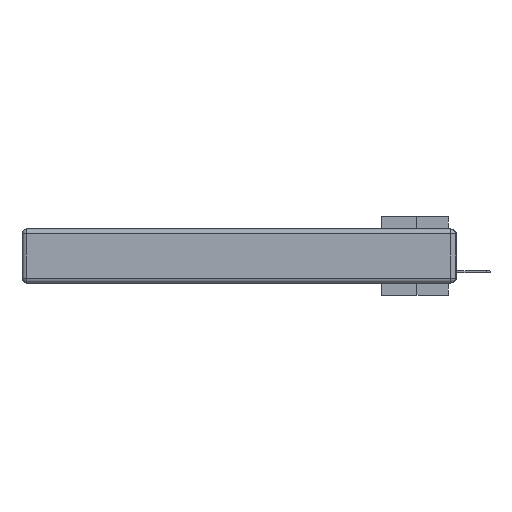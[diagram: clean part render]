
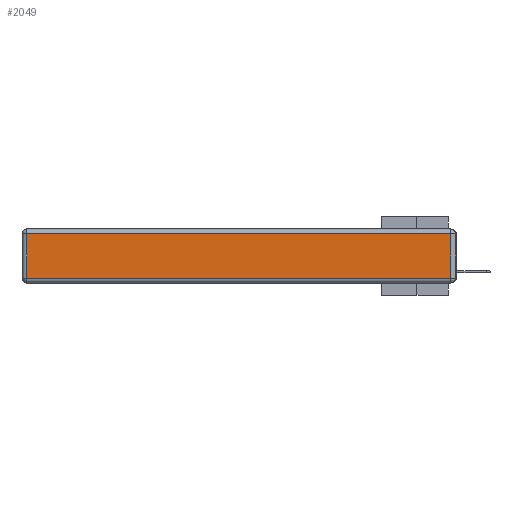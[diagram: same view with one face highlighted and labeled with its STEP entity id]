
A CAD part, left-side view. The second image highlights one B-rep face of the part: STEP entity #2049.
In plain terms, the highlighted planar face has unit normal (-1, 0, 0).
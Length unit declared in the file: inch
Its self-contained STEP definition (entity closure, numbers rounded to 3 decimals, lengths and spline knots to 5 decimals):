
#412 = DIRECTION ( 'NONE',  ( 0., 1., 0. ) ) ;
#1470 = LINE ( 'NONE', #4360, #27124 ) ;
#2049 = ADVANCED_FACE ( 'NONE', ( #32304 ), #18576, .T. ) ;
#3308 = CARTESIAN_POINT ( 'NONE',  ( 0., 2.75, -0.03 ) ) ;
#3401 = EDGE_CURVE ( 'NONE', #28576, #4793, #19665, .T. ) ;
#3579 = ORIENTED_EDGE ( 'NONE', *, *, #27160, .T. ) ;
#4360 = CARTESIAN_POINT ( 'NONE',  ( 0., 0.03, -0.343 ) ) ;
#4760 = CARTESIAN_POINT ( 'NONE',  ( 0., 0., -0.343 ) ) ;
#4793 = VERTEX_POINT ( 'NONE', #31206 ) ;
#6296 = EDGE_LOOP ( 'NONE', ( #3579, #31972, #23948, #17281 ) ) ;
#6326 = DIRECTION ( 'NONE',  ( 0., 0., 1. ) ) ;
#8368 = CARTESIAN_POINT ( 'NONE',  ( 0., 2.72, -0.313 ) ) ;
#8478 = EDGE_CURVE ( 'NONE', #4793, #15131, #19443, .T. ) ;
#9550 = CARTESIAN_POINT ( 'NONE',  ( 0., 0., -0.313 ) ) ;
#13141 = DIRECTION ( 'NONE',  ( -1., 0., 0. ) ) ;
#13359 = VERTEX_POINT ( 'NONE', #27454 ) ;
#15131 = VERTEX_POINT ( 'NONE', #8368 ) ;
#15206 = DIRECTION ( 'NONE',  ( 0., -1., 0. ) ) ;
#15406 = VECTOR ( 'NONE', #33001, 39.37008 ) ;
#17281 = ORIENTED_EDGE ( 'NONE', *, *, #8478, .T. ) ;
#18576 = PLANE ( 'NONE',  #34975 ) ;
#18721 = CARTESIAN_POINT ( 'NONE',  ( 0., 2.72, -0.343 ) ) ;
#19443 = LINE ( 'NONE', #18721, #15406 ) ;
#19665 = LINE ( 'NONE', #3308, #25637 ) ;
#20035 = VECTOR ( 'NONE', #15206, 39.37008 ) ;
#21422 = DIRECTION ( 'NONE',  ( 0., 0., 1. ) ) ;
#23948 = ORIENTED_EDGE ( 'NONE', *, *, #3401, .T. ) ;
#25637 = VECTOR ( 'NONE', #412, 39.37008 ) ;
#25700 = LINE ( 'NONE', #9550, #20035 ) ;
#27124 = VECTOR ( 'NONE', #21422, 39.37008 ) ;
#27153 = CARTESIAN_POINT ( 'NONE',  ( 0., 0.03, -0.03 ) ) ;
#27160 = EDGE_CURVE ( 'NONE', #15131, #13359, #25700, .T. ) ;
#27454 = CARTESIAN_POINT ( 'NONE',  ( 0., 0.03, -0.313 ) ) ;
#28576 = VERTEX_POINT ( 'NONE', #27153 ) ;
#31206 = CARTESIAN_POINT ( 'NONE',  ( 0., 2.72, -0.03 ) ) ;
#31457 = EDGE_CURVE ( 'NONE', #13359, #28576, #1470, .T. ) ;
#31972 = ORIENTED_EDGE ( 'NONE', *, *, #31457, .T. ) ;
#32304 = FACE_OUTER_BOUND ( 'NONE', #6296, .T. ) ;
#33001 = DIRECTION ( 'NONE',  ( 0., 0., -1. ) ) ;
#34975 = AXIS2_PLACEMENT_3D ( 'NONE', #4760, #13141, #6326 ) ;
